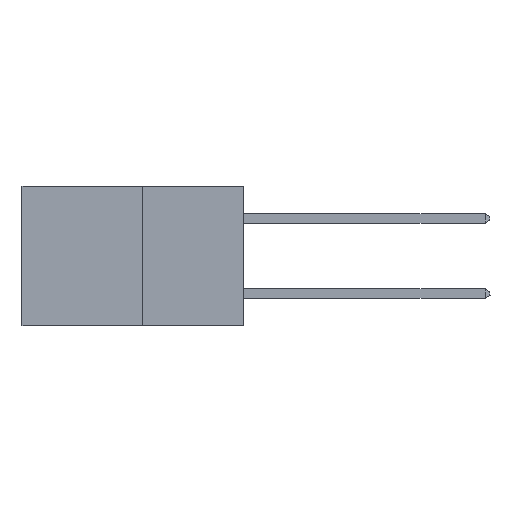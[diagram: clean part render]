
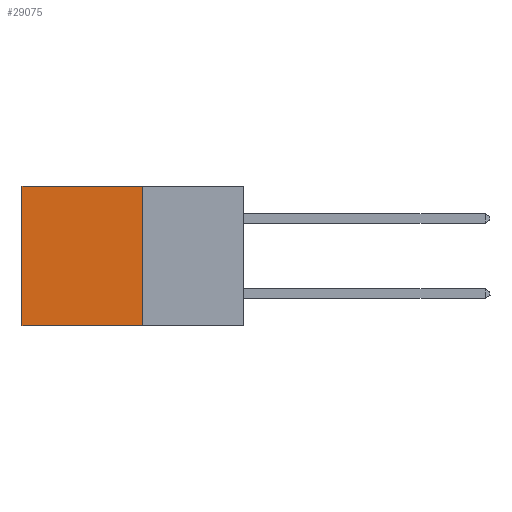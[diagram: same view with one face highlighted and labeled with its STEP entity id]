
A CAD part, left-side view. The second image highlights one B-rep face of the part: STEP entity #29075.
In plain terms, the highlighted planar face has unit normal (-1, 0, 0).
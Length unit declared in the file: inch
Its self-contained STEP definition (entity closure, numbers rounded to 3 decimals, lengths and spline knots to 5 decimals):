
#1307 = DIRECTION ( 'NONE',  ( 0., 0., -1. ) ) ;
#2125 = ORIENTED_EDGE ( 'NONE', *, *, #11415, .F. ) ;
#2222 = VERTEX_POINT ( 'NONE', #16156 ) ;
#2954 = EDGE_LOOP ( 'NONE', ( #17636, #2125, #16230, #27910 ) ) ;
#3234 = EDGE_CURVE ( 'NONE', #27181, #26392, #15541, .T. ) ;
#3333 = FACE_OUTER_BOUND ( 'NONE', #2954, .T. ) ;
#3700 = CARTESIAN_POINT ( 'NONE',  ( 0.277, 0.59, -0.37 ) ) ;
#3933 = VECTOR ( 'NONE', #25338, 39.37008 ) ;
#5676 = VERTEX_POINT ( 'NONE', #21591 ) ;
#5764 = VECTOR ( 'NONE', #17783, 39.37008 ) ;
#5957 = DIRECTION ( 'NONE',  ( 0., 0., -1. ) ) ;
#7003 = CARTESIAN_POINT ( 'NONE',  ( 0.277, 0.27, -0.37 ) ) ;
#9155 = DIRECTION ( 'NONE',  ( 0., 0., -1. ) ) ;
#9283 = VECTOR ( 'NONE', #5957, 39.37008 ) ;
#10266 = LINE ( 'NONE', #18446, #3933 ) ;
#11347 = LINE ( 'NONE', #29282, #5764 ) ;
#11415 = EDGE_CURVE ( 'NONE', #26392, #2222, #10266, .T. ) ;
#11446 = PLANE ( 'NONE',  #12562 ) ;
#11888 = CARTESIAN_POINT ( 'NONE',  ( 0.277, 0.27, 0. ) ) ;
#12562 = AXIS2_PLACEMENT_3D ( 'NONE', #20788, #23119, #9155 ) ;
#13679 = EDGE_CURVE ( 'NONE', #5676, #2222, #16290, .T. ) ;
#15541 = LINE ( 'NONE', #7003, #9283 ) ;
#16156 = CARTESIAN_POINT ( 'NONE',  ( 0.277, 0.59, -0.37 ) ) ;
#16230 = ORIENTED_EDGE ( 'NONE', *, *, #3234, .F. ) ;
#16290 = LINE ( 'NONE', #3700, #27854 ) ;
#17636 = ORIENTED_EDGE ( 'NONE', *, *, #13679, .T. ) ;
#17783 = DIRECTION ( 'NONE',  ( 0., 1., 0. ) ) ;
#18446 = CARTESIAN_POINT ( 'NONE',  ( 0.277, 0.27, -0.37 ) ) ;
#20788 = CARTESIAN_POINT ( 'NONE',  ( 0.277, 0.27, -0.37 ) ) ;
#21591 = CARTESIAN_POINT ( 'NONE',  ( 0.277, 0.59, 0. ) ) ;
#23119 = DIRECTION ( 'NONE',  ( 1., 0., 0. ) ) ;
#24876 = EDGE_CURVE ( 'NONE', #27181, #5676, #11347, .T. ) ;
#25338 = DIRECTION ( 'NONE',  ( 0., 1., 0. ) ) ;
#25417 = CARTESIAN_POINT ( 'NONE',  ( 0.277, 0.27, -0.37 ) ) ;
#26392 = VERTEX_POINT ( 'NONE', #25417 ) ;
#27181 = VERTEX_POINT ( 'NONE', #11888 ) ;
#27854 = VECTOR ( 'NONE', #1307, 39.37008 ) ;
#27910 = ORIENTED_EDGE ( 'NONE', *, *, #24876, .T. ) ;
#29075 = ADVANCED_FACE ( 'NONE', ( #3333 ), #11446, .F. ) ;
#29282 = CARTESIAN_POINT ( 'NONE',  ( 0.277, 0.27, 0. ) ) ;
